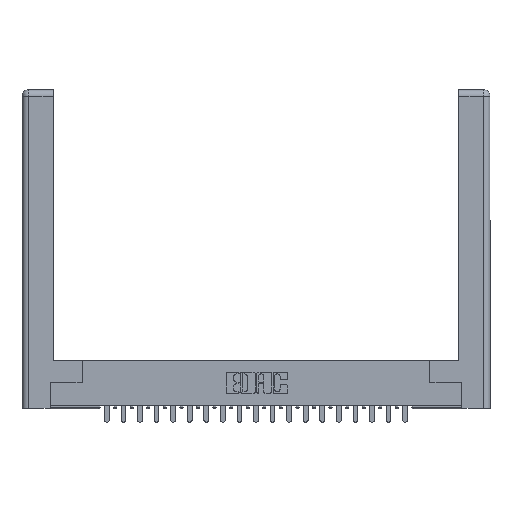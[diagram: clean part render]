
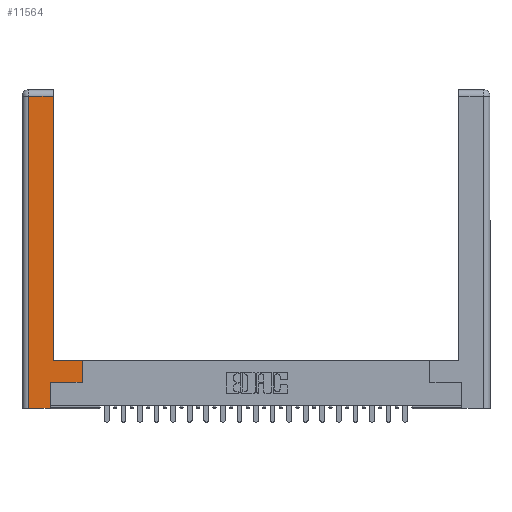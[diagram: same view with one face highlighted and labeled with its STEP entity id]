
A CAD part, top view. The second image highlights one B-rep face of the part: STEP entity #11564.
In plain terms, the highlighted planar face has unit normal (0, 0, 1).
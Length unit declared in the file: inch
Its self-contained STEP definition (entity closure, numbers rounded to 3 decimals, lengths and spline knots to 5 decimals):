
#828 = VECTOR ( 'NONE', #4879, 39.37008 ) ;
#1111 = EDGE_CURVE ( 'NONE', #5436, #11771, #1152, .T. ) ;
#1152 = LINE ( 'NONE', #22139, #16389 ) ;
#1361 = VERTEX_POINT ( 'NONE', #13110 ) ;
#1710 = EDGE_CURVE ( 'NONE', #18675, #5436, #16672, .T. ) ;
#2165 = AXIS2_PLACEMENT_3D ( 'NONE', #17142, #7226, #17563 ) ;
#2302 = VECTOR ( 'NONE', #3247, 39.37008 ) ;
#2526 = CARTESIAN_POINT ( 'NONE',  ( 0.295, 0.45, 0. ) ) ;
#2698 = ORIENTED_EDGE ( 'NONE', *, *, #23123, .T. ) ;
#2758 = CARTESIAN_POINT ( 'NONE',  ( 0.0615, 2.94, 0. ) ) ;
#2764 = CARTESIAN_POINT ( 'NONE',  ( 0.295, 0.45, 0. ) ) ;
#3134 = LINE ( 'NONE', #2758, #5648 ) ;
#3247 = DIRECTION ( 'NONE',  ( 0., 1., 0. ) ) ;
#4004 = ORIENTED_EDGE ( 'NONE', *, *, #1710, .T. ) ;
#4251 = DIRECTION ( 'NONE',  ( 0., 1., 0. ) ) ;
#4676 = CARTESIAN_POINT ( 'NONE',  ( 0.565, 0.245, 0. ) ) ;
#4879 = DIRECTION ( 'NONE',  ( -1., 0., 0. ) ) ;
#5436 = VERTEX_POINT ( 'NONE', #11838 ) ;
#5648 = VECTOR ( 'NONE', #10527, 39.37008 ) ;
#7226 = DIRECTION ( 'NONE',  ( 0., 0., -1. ) ) ;
#8189 = VECTOR ( 'NONE', #13242, 39.37008 ) ;
#8279 = CARTESIAN_POINT ( 'NONE',  ( 0.0615, 0., 0. ) ) ;
#8411 = VERTEX_POINT ( 'NONE', #2526 ) ;
#8688 = LINE ( 'NONE', #17193, #19261 ) ;
#9061 = EDGE_CURVE ( 'NONE', #15211, #1361, #3134, .T. ) ;
#9974 = FACE_OUTER_BOUND ( 'NONE', #14684, .T. ) ;
#10527 = DIRECTION ( 'NONE',  ( -1., 0., 0. ) ) ;
#11057 = VECTOR ( 'NONE', #11304, 39.37008 ) ;
#11304 = DIRECTION ( 'NONE',  ( 0., 1., 0. ) ) ;
#11350 = DIRECTION ( 'NONE',  ( 1., 0., 0. ) ) ;
#11564 = ADVANCED_FACE ( 'NONE', ( #9974 ), #25112, .F. ) ;
#11771 = VERTEX_POINT ( 'NONE', #22021 ) ;
#11838 = CARTESIAN_POINT ( 'NONE',  ( 0.565, 0.245, 0. ) ) ;
#12129 = EDGE_CURVE ( 'NONE', #24559, #24026, #8688, .T. ) ;
#12279 = LINE ( 'NONE', #23065, #2302 ) ;
#13110 = CARTESIAN_POINT ( 'NONE',  ( 0.0615, 2.94, 0. ) ) ;
#13242 = DIRECTION ( 'NONE',  ( 0., -1., 0. ) ) ;
#14684 = EDGE_LOOP ( 'NONE', ( #18508, #16423, #2698, #17316, #18398, #4004, #16349, #22631 ) ) ;
#15211 = VERTEX_POINT ( 'NONE', #22743 ) ;
#15834 = CARTESIAN_POINT ( 'NONE',  ( 0.265, 0.245, 0. ) ) ;
#16076 = EDGE_CURVE ( 'NONE', #24026, #18675, #22296, .T. ) ;
#16228 = EDGE_CURVE ( 'NONE', #8411, #15211, #12279, .T. ) ;
#16349 = ORIENTED_EDGE ( 'NONE', *, *, #1111, .T. ) ;
#16389 = VECTOR ( 'NONE', #4251, 39.37008 ) ;
#16423 = ORIENTED_EDGE ( 'NONE', *, *, #9061, .T. ) ;
#16672 = LINE ( 'NONE', #4676, #20117 ) ;
#17142 = CARTESIAN_POINT ( 'NONE',  ( 0., 0., 0. ) ) ;
#17193 = CARTESIAN_POINT ( 'NONE',  ( 0.265, 0., 0. ) ) ;
#17316 = ORIENTED_EDGE ( 'NONE', *, *, #12129, .T. ) ;
#17563 = DIRECTION ( 'NONE',  ( -1., 0., 0. ) ) ;
#18398 = ORIENTED_EDGE ( 'NONE', *, *, #16076, .T. ) ;
#18508 = ORIENTED_EDGE ( 'NONE', *, *, #16228, .T. ) ;
#18546 = CARTESIAN_POINT ( 'NONE',  ( 0.265, 0., 0. ) ) ;
#18675 = VERTEX_POINT ( 'NONE', #15834 ) ;
#19261 = VECTOR ( 'NONE', #11350, 39.37008 ) ;
#20117 = VECTOR ( 'NONE', #20160, 39.37008 ) ;
#20160 = DIRECTION ( 'NONE',  ( 1., 0., 0. ) ) ;
#20485 = CARTESIAN_POINT ( 'NONE',  ( 0.0615, 0., 0. ) ) ;
#20912 = EDGE_CURVE ( 'NONE', #11771, #8411, #22667, .T. ) ;
#21574 = LINE ( 'NONE', #20485, #8189 ) ;
#22021 = CARTESIAN_POINT ( 'NONE',  ( 0.565, 0.45, 0. ) ) ;
#22139 = CARTESIAN_POINT ( 'NONE',  ( 0.565, 0.45, 0. ) ) ;
#22296 = LINE ( 'NONE', #25562, #11057 ) ;
#22631 = ORIENTED_EDGE ( 'NONE', *, *, #20912, .T. ) ;
#22667 = LINE ( 'NONE', #2764, #828 ) ;
#22743 = CARTESIAN_POINT ( 'NONE',  ( 0.295, 2.94, 0. ) ) ;
#23065 = CARTESIAN_POINT ( 'NONE',  ( 0.295, 3., 0. ) ) ;
#23123 = EDGE_CURVE ( 'NONE', #1361, #24559, #21574, .T. ) ;
#24026 = VERTEX_POINT ( 'NONE', #18546 ) ;
#24559 = VERTEX_POINT ( 'NONE', #8279 ) ;
#25112 = PLANE ( 'NONE',  #2165 ) ;
#25562 = CARTESIAN_POINT ( 'NONE',  ( 0.265, 0.245, 0. ) ) ;
